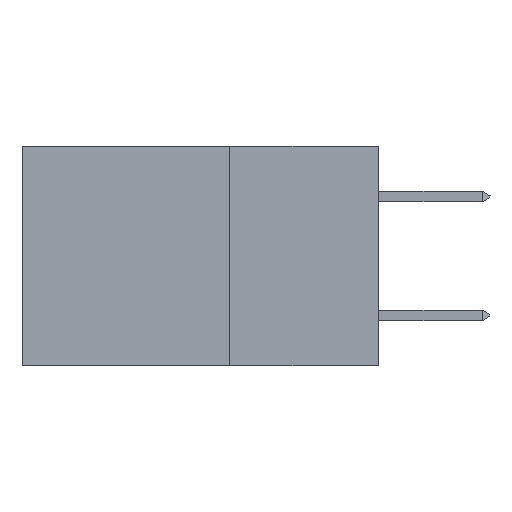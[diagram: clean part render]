
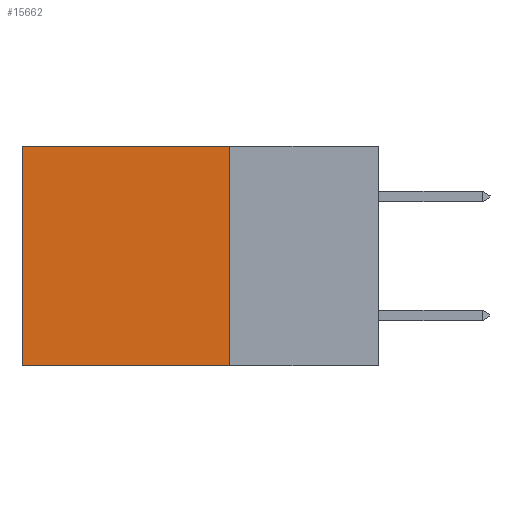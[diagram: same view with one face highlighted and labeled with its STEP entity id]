
A CAD part, left-side view. The second image highlights one B-rep face of the part: STEP entity #15662.
In plain terms, the highlighted planar face has unit normal (-1, 0, 0).
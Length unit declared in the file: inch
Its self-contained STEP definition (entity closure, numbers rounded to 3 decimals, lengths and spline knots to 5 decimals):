
#790 = DIRECTION ( 'NONE',  ( 0., 0., -1. ) ) ;
#1647 = LINE ( 'NONE', #6100, #17176 ) ;
#3113 = DIRECTION ( 'NONE',  ( 0., 1., 0. ) ) ;
#3703 = DIRECTION ( 'NONE',  ( 0., 0., -1. ) ) ;
#5817 = CARTESIAN_POINT ( 'NONE',  ( 0.2615, 0.6, 0. ) ) ;
#5965 = DIRECTION ( 'NONE',  ( 0., 0., -1. ) ) ;
#6100 = CARTESIAN_POINT ( 'NONE',  ( 0.2615, 0.25, -0.37 ) ) ;
#6382 = FACE_OUTER_BOUND ( 'NONE', #21352, .T. ) ;
#7333 = CARTESIAN_POINT ( 'NONE',  ( 0.2615, 0.25, 0. ) ) ;
#9400 = VECTOR ( 'NONE', #3113, 39.37008 ) ;
#9834 = CARTESIAN_POINT ( 'NONE',  ( 0.2615, 0.25, -0.37 ) ) ;
#10209 = AXIS2_PLACEMENT_3D ( 'NONE', #19743, #10260, #790 ) ;
#10260 = DIRECTION ( 'NONE',  ( 1., 0., 0. ) ) ;
#10973 = CARTESIAN_POINT ( 'NONE',  ( 0.2615, 0.25, 0. ) ) ;
#11365 = VECTOR ( 'NONE', #3703, 39.37008 ) ;
#11633 = EDGE_CURVE ( 'NONE', #18589, #17379, #1647, .T. ) ;
#13024 = CARTESIAN_POINT ( 'NONE',  ( 0.2615, 0.25, -0.37 ) ) ;
#13353 = LINE ( 'NONE', #9834, #15782 ) ;
#13727 = DIRECTION ( 'NONE',  ( 0., 1., 0. ) ) ;
#13860 = EDGE_CURVE ( 'NONE', #22399, #17379, #16930, .T. ) ;
#14497 = ORIENTED_EDGE ( 'NONE', *, *, #16346, .T. ) ;
#15662 = ADVANCED_FACE ( 'NONE', ( #6382 ), #21733, .F. ) ;
#15782 = VECTOR ( 'NONE', #5965, 39.37008 ) ;
#15993 = EDGE_CURVE ( 'NONE', #17622, #18589, #13353, .T. ) ;
#16346 = EDGE_CURVE ( 'NONE', #17622, #22399, #22054, .T. ) ;
#16531 = ORIENTED_EDGE ( 'NONE', *, *, #11633, .F. ) ;
#16930 = LINE ( 'NONE', #17046, #11365 ) ;
#17046 = CARTESIAN_POINT ( 'NONE',  ( 0.2615, 0.6, -0.37 ) ) ;
#17176 = VECTOR ( 'NONE', #13727, 39.37008 ) ;
#17379 = VERTEX_POINT ( 'NONE', #23060 ) ;
#17622 = VERTEX_POINT ( 'NONE', #7333 ) ;
#18589 = VERTEX_POINT ( 'NONE', #13024 ) ;
#19743 = CARTESIAN_POINT ( 'NONE',  ( 0.2615, 0.25, -0.37 ) ) ;
#20797 = ORIENTED_EDGE ( 'NONE', *, *, #15993, .F. ) ;
#21352 = EDGE_LOOP ( 'NONE', ( #23355, #16531, #20797, #14497 ) ) ;
#21733 = PLANE ( 'NONE',  #10209 ) ;
#22054 = LINE ( 'NONE', #10973, #9400 ) ;
#22399 = VERTEX_POINT ( 'NONE', #5817 ) ;
#23060 = CARTESIAN_POINT ( 'NONE',  ( 0.2615, 0.6, -0.37 ) ) ;
#23355 = ORIENTED_EDGE ( 'NONE', *, *, #13860, .T. ) ;
